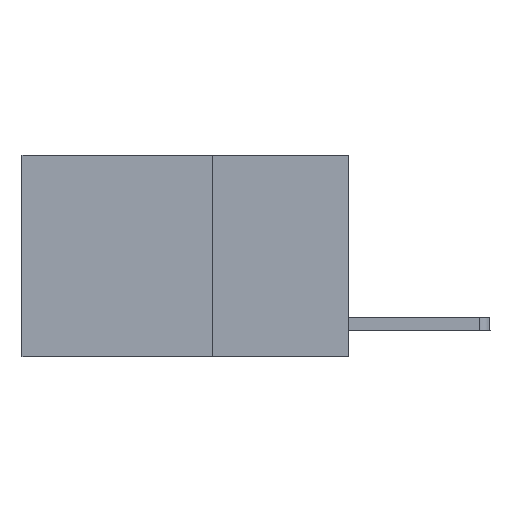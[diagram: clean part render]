
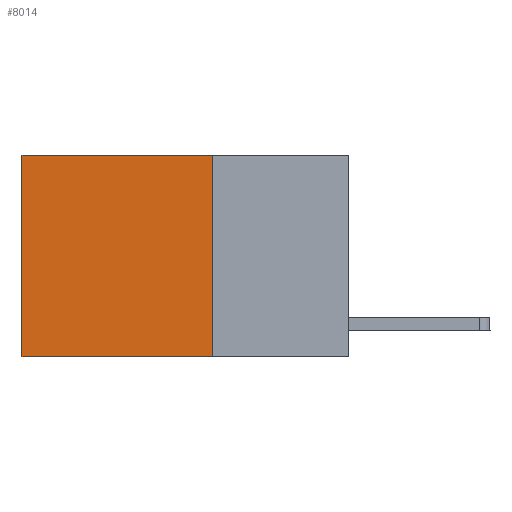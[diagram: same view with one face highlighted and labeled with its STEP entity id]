
A CAD part, left-side view. The second image highlights one B-rep face of the part: STEP entity #8014.
In plain terms, the highlighted planar face has unit normal (-1, 0, 0).
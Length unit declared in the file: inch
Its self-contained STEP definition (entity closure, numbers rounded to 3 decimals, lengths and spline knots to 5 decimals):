
#156 = CARTESIAN_POINT ( 'NONE',  ( 0.2625, 0.25, 0. ) ) ;
#653 = FACE_OUTER_BOUND ( 'NONE', #7013, .T. ) ;
#756 = DIRECTION ( 'NONE',  ( 0., 0., -1. ) ) ;
#960 = VECTOR ( 'NONE', #4213, 39.37008 ) ;
#1626 = CARTESIAN_POINT ( 'NONE',  ( 0.2625, 0.6, 0. ) ) ;
#1663 = CARTESIAN_POINT ( 'NONE',  ( 0.2625, 0.25, 0. ) ) ;
#2189 = CARTESIAN_POINT ( 'NONE',  ( 0.2625, 0.6, -0.37 ) ) ;
#2220 = EDGE_CURVE ( 'NONE', #10385, #3262, #9212, .T. ) ;
#2289 = CARTESIAN_POINT ( 'NONE',  ( 0.2625, 0.25, -0.37 ) ) ;
#2474 = ORIENTED_EDGE ( 'NONE', *, *, #4362, .T. ) ;
#2496 = VECTOR ( 'NONE', #7840, 39.37008 ) ;
#3144 = EDGE_CURVE ( 'NONE', #10225, #7127, #5686, .T. ) ;
#3262 = VERTEX_POINT ( 'NONE', #7689 ) ;
#3385 = EDGE_CURVE ( 'NONE', #3262, #7127, #9647, .T. ) ;
#4213 = DIRECTION ( 'NONE',  ( 0., 0., -1. ) ) ;
#4362 = EDGE_CURVE ( 'NONE', #10385, #10225, #5853, .T. ) ;
#4755 = VECTOR ( 'NONE', #7377, 39.37008 ) ;
#4800 = CARTESIAN_POINT ( 'NONE',  ( 0.2625, 0.25, 0. ) ) ;
#5295 = ORIENTED_EDGE ( 'NONE', *, *, #3385, .F. ) ;
#5383 = ORIENTED_EDGE ( 'NONE', *, *, #3144, .T. ) ;
#5686 = LINE ( 'NONE', #1626, #9311 ) ;
#5853 = LINE ( 'NONE', #156, #4755 ) ;
#6054 = AXIS2_PLACEMENT_3D ( 'NONE', #4800, #9627, #756 ) ;
#6690 = CARTESIAN_POINT ( 'NONE',  ( 0.2625, 0.25, 0. ) ) ;
#7013 = EDGE_LOOP ( 'NONE', ( #5383, #5295, #8911, #2474 ) ) ;
#7127 = VERTEX_POINT ( 'NONE', #2189 ) ;
#7374 = DIRECTION ( 'NONE',  ( 0., 0., -1. ) ) ;
#7377 = DIRECTION ( 'NONE',  ( 0., 1., 0. ) ) ;
#7689 = CARTESIAN_POINT ( 'NONE',  ( 0.2625, 0.25, -0.37 ) ) ;
#7840 = DIRECTION ( 'NONE',  ( 0., 1., 0. ) ) ;
#8014 = ADVANCED_FACE ( 'NONE', ( #653 ), #9581, .F. ) ;
#8746 = CARTESIAN_POINT ( 'NONE',  ( 0.2625, 0.6, 0. ) ) ;
#8911 = ORIENTED_EDGE ( 'NONE', *, *, #2220, .F. ) ;
#9212 = LINE ( 'NONE', #6690, #960 ) ;
#9311 = VECTOR ( 'NONE', #7374, 39.37008 ) ;
#9581 = PLANE ( 'NONE',  #6054 ) ;
#9627 = DIRECTION ( 'NONE',  ( 1., 0., 0. ) ) ;
#9647 = LINE ( 'NONE', #2289, #2496 ) ;
#10225 = VERTEX_POINT ( 'NONE', #8746 ) ;
#10385 = VERTEX_POINT ( 'NONE', #1663 ) ;
